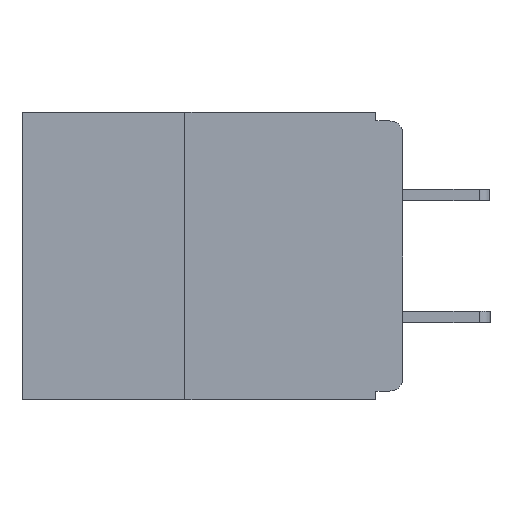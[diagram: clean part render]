
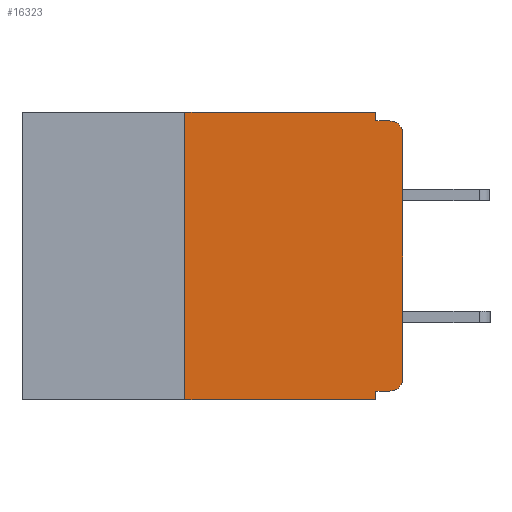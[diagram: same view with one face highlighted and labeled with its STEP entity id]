
A CAD part, left-side view. The second image highlights one B-rep face of the part: STEP entity #16323.
In plain terms, the highlighted planar face has unit normal (-1, 0, 0).
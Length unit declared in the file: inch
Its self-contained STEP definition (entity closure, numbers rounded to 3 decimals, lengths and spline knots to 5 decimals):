
#128 = CIRCLE ( 'NONE', #3215, 0.015 ) ;
#1062 = VERTEX_POINT ( 'NONE', #25409 ) ;
#1307 = EDGE_CURVE ( 'NONE', #23585, #24219, #23369, .T. ) ;
#2198 = ORIENTED_EDGE ( 'NONE', *, *, #5809, .F. ) ;
#2251 = DIRECTION ( 'NONE',  ( 0., 0., -1. ) ) ;
#3196 = ORIENTED_EDGE ( 'NONE', *, *, #11412, .T. ) ;
#3215 = AXIS2_PLACEMENT_3D ( 'NONE', #22273, #22261, #22234 ) ;
#3675 = VERTEX_POINT ( 'NONE', #25719 ) ;
#4310 = VECTOR ( 'NONE', #16283, 39.37008 ) ;
#4463 = PLANE ( 'NONE',  #24815 ) ;
#5009 = FACE_OUTER_BOUND ( 'NONE', #15827, .T. ) ;
#5418 = ORIENTED_EDGE ( 'NONE', *, *, #1307, .F. ) ;
#5522 = VECTOR ( 'NONE', #14113, 39.37008 ) ;
#5809 = EDGE_CURVE ( 'NONE', #24219, #6693, #21574, .T. ) ;
#5862 = CARTESIAN_POINT ( 'NONE',  ( 0., 0., -0.305 ) ) ;
#5930 = AXIS2_PLACEMENT_3D ( 'NONE', #11320, #25227, #13300 ) ;
#6362 = VECTOR ( 'NONE', #19068, 39.37008 ) ;
#6511 = CARTESIAN_POINT ( 'NONE',  ( 0., 0.437, 0. ) ) ;
#6564 = CARTESIAN_POINT ( 'NONE',  ( 0., 0., -0.025 ) ) ;
#6576 = CARTESIAN_POINT ( 'NONE',  ( 0., 0.031, -0.01 ) ) ;
#6693 = VERTEX_POINT ( 'NONE', #21256 ) ;
#6740 = ORIENTED_EDGE ( 'NONE', *, *, #16122, .F. ) ;
#7106 = CARTESIAN_POINT ( 'NONE',  ( 0., 0.031, -0.32 ) ) ;
#7138 = CARTESIAN_POINT ( 'NONE',  ( 0., 0.015, -0.32 ) ) ;
#7196 = EDGE_CURVE ( 'NONE', #3675, #6693, #23405, .T. ) ;
#7272 = EDGE_CURVE ( 'NONE', #21329, #1062, #12163, .T. ) ;
#7411 = LINE ( 'NONE', #21631, #18070 ) ;
#7819 = ORIENTED_EDGE ( 'NONE', *, *, #19469, .T. ) ;
#7838 = ORIENTED_EDGE ( 'NONE', *, *, #7196, .T. ) ;
#7924 = DIRECTION ( 'NONE',  ( 0., -1., 0. ) ) ;
#8544 = DIRECTION ( 'NONE',  ( 1., 0., 0. ) ) ;
#8547 = EDGE_CURVE ( 'NONE', #3675, #21329, #7411, .T. ) ;
#9433 = VECTOR ( 'NONE', #7924, 39.37008 ) ;
#9491 = ORIENTED_EDGE ( 'NONE', *, *, #15245, .F. ) ;
#9768 = ORIENTED_EDGE ( 'NONE', *, *, #10515, .T. ) ;
#10515 = EDGE_CURVE ( 'NONE', #25093, #16937, #16407, .T. ) ;
#11320 = CARTESIAN_POINT ( 'NONE',  ( 0., 0.015, -0.025 ) ) ;
#11412 = EDGE_CURVE ( 'NONE', #23585, #25093, #128, .T. ) ;
#12163 = LINE ( 'NONE', #14217, #5522 ) ;
#12781 = VECTOR ( 'NONE', #15874, 39.37008 ) ;
#13300 = DIRECTION ( 'NONE',  ( 0., 0., -1. ) ) ;
#13408 = DIRECTION ( 'NONE',  ( 0., 1., 0. ) ) ;
#14113 = DIRECTION ( 'NONE',  ( 0., -1., 0. ) ) ;
#14217 = CARTESIAN_POINT ( 'NONE',  ( 0., 0.437, 0. ) ) ;
#14291 = ORIENTED_EDGE ( 'NONE', *, *, #8547, .F. ) ;
#15215 = CARTESIAN_POINT ( 'NONE',  ( 0., 0.437, -0.33 ) ) ;
#15245 = EDGE_CURVE ( 'NONE', #1062, #22224, #25049, .T. ) ;
#15706 = VECTOR ( 'NONE', #2251, 39.37008 ) ;
#15827 = EDGE_LOOP ( 'NONE', ( #9768, #7819, #6740, #9491, #24611, #14291, #7838, #2198, #5418, #3196 ) ) ;
#15874 = DIRECTION ( 'NONE',  ( 0., -1., 0. ) ) ;
#16122 = EDGE_CURVE ( 'NONE', #22224, #22614, #21346, .T. ) ;
#16267 = CARTESIAN_POINT ( 'NONE',  ( 0., 0.031, -0.33 ) ) ;
#16283 = DIRECTION ( 'NONE',  ( 0., 0., -1. ) ) ;
#16323 = ADVANCED_FACE ( 'NONE', ( #5009 ), #4463, .F. ) ;
#16407 = LINE ( 'NONE', #19123, #6362 ) ;
#16937 = VERTEX_POINT ( 'NONE', #6564 ) ;
#18070 = VECTOR ( 'NONE', #25242, 39.37008 ) ;
#18418 = CARTESIAN_POINT ( 'NONE',  ( 0., 0.031, 0. ) ) ;
#19068 = DIRECTION ( 'NONE',  ( 0., 0., 1. ) ) ;
#19123 = CARTESIAN_POINT ( 'NONE',  ( 0., 0., 0. ) ) ;
#19418 = CARTESIAN_POINT ( 'NONE',  ( 0., 0., -0.32 ) ) ;
#19469 = EDGE_CURVE ( 'NONE', #16937, #22614, #25141, .T. ) ;
#20223 = CARTESIAN_POINT ( 'NONE',  ( 0., 0.015, -0.01 ) ) ;
#21256 = CARTESIAN_POINT ( 'NONE',  ( 0., 0.031, -0.33 ) ) ;
#21329 = VERTEX_POINT ( 'NONE', #23790 ) ;
#21346 = LINE ( 'NONE', #21920, #9433 ) ;
#21574 = LINE ( 'NONE', #16267, #4310 ) ;
#21631 = CARTESIAN_POINT ( 'NONE',  ( 0., 0.25, -0.33 ) ) ;
#21920 = CARTESIAN_POINT ( 'NONE',  ( 0., 0., -0.01 ) ) ;
#22224 = VERTEX_POINT ( 'NONE', #6576 ) ;
#22234 = DIRECTION ( 'NONE',  ( 0., 0., -1. ) ) ;
#22261 = DIRECTION ( 'NONE',  ( -1., 0., 0. ) ) ;
#22273 = CARTESIAN_POINT ( 'NONE',  ( 0., 0.015, -0.305 ) ) ;
#22530 = DIRECTION ( 'NONE',  ( 0., 0., -1. ) ) ;
#22614 = VERTEX_POINT ( 'NONE', #20223 ) ;
#22770 = VECTOR ( 'NONE', #13408, 39.37008 ) ;
#23369 = LINE ( 'NONE', #19418, #22770 ) ;
#23405 = LINE ( 'NONE', #15215, #12781 ) ;
#23585 = VERTEX_POINT ( 'NONE', #7138 ) ;
#23790 = CARTESIAN_POINT ( 'NONE',  ( 0., 0.25, 0. ) ) ;
#24219 = VERTEX_POINT ( 'NONE', #7106 ) ;
#24611 = ORIENTED_EDGE ( 'NONE', *, *, #7272, .F. ) ;
#24815 = AXIS2_PLACEMENT_3D ( 'NONE', #6511, #8544, #22530 ) ;
#25049 = LINE ( 'NONE', #18418, #15706 ) ;
#25093 = VERTEX_POINT ( 'NONE', #5862 ) ;
#25141 = CIRCLE ( 'NONE', #5930, 0.015 ) ;
#25227 = DIRECTION ( 'NONE',  ( -1., 0., 0. ) ) ;
#25242 = DIRECTION ( 'NONE',  ( 0., 0., 1. ) ) ;
#25409 = CARTESIAN_POINT ( 'NONE',  ( 0., 0.031, 0. ) ) ;
#25719 = CARTESIAN_POINT ( 'NONE',  ( 0., 0.25, -0.33 ) ) ;
